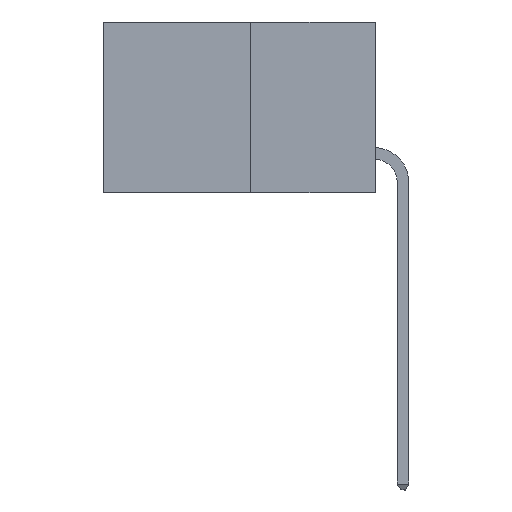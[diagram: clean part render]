
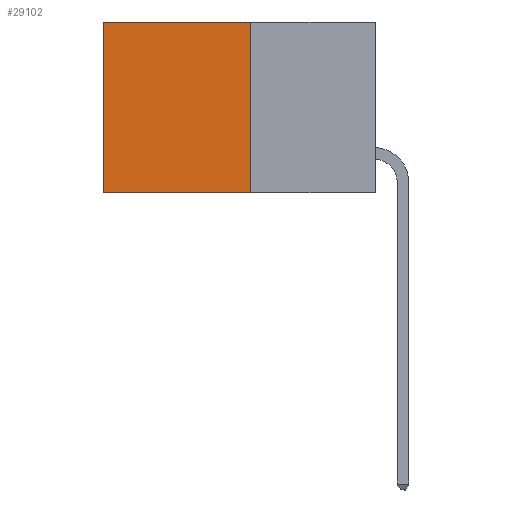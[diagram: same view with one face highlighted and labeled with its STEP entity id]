
A CAD part, left-side view. The second image highlights one B-rep face of the part: STEP entity #29102.
In plain terms, the highlighted planar face has unit normal (-1, 0, 0).
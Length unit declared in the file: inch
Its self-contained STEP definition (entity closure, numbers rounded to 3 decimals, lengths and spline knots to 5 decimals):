
#975 = VECTOR ( 'NONE', #7875, 39.37008 ) ;
#1063 = CARTESIAN_POINT ( 'NONE',  ( 0.277, 0.59, -0.37 ) ) ;
#1891 = CARTESIAN_POINT ( 'NONE',  ( 0.277, 0.27, -0.37 ) ) ;
#3534 = CARTESIAN_POINT ( 'NONE',  ( 0.277, 0.27, 0. ) ) ;
#4272 = DIRECTION ( 'NONE',  ( 1., 0., 0. ) ) ;
#5328 = FACE_OUTER_BOUND ( 'NONE', #15269, .T. ) ;
#5579 = EDGE_CURVE ( 'NONE', #9279, #24971, #29126, .T. ) ;
#6140 = EDGE_CURVE ( 'NONE', #8766, #24971, #7004, .T. ) ;
#6614 = CARTESIAN_POINT ( 'NONE',  ( 0.277, 0.59, -0.37 ) ) ;
#6671 = VECTOR ( 'NONE', #14795, 39.37008 ) ;
#7004 = LINE ( 'NONE', #19068, #975 ) ;
#7298 = CARTESIAN_POINT ( 'NONE',  ( 0.277, 0.59, 0. ) ) ;
#7875 = DIRECTION ( 'NONE',  ( 0., 1., 0. ) ) ;
#8153 = ORIENTED_EDGE ( 'NONE', *, *, #5579, .T. ) ;
#8766 = VERTEX_POINT ( 'NONE', #27818 ) ;
#9254 = ORIENTED_EDGE ( 'NONE', *, *, #22810, .T. ) ;
#9275 = CARTESIAN_POINT ( 'NONE',  ( 0.277, 0.27, -0.37 ) ) ;
#9279 = VERTEX_POINT ( 'NONE', #7298 ) ;
#11557 = DIRECTION ( 'NONE',  ( 0., 0., -1. ) ) ;
#14795 = DIRECTION ( 'NONE',  ( 0., 1., 0. ) ) ;
#15269 = EDGE_LOOP ( 'NONE', ( #8153, #20236, #20645, #9254 ) ) ;
#16528 = VECTOR ( 'NONE', #21336, 39.37008 ) ;
#17738 = CARTESIAN_POINT ( 'NONE',  ( 0.277, 0.27, 0. ) ) ;
#19068 = CARTESIAN_POINT ( 'NONE',  ( 0.277, 0.27, -0.37 ) ) ;
#20004 = DIRECTION ( 'NONE',  ( 0., 0., -1. ) ) ;
#20236 = ORIENTED_EDGE ( 'NONE', *, *, #6140, .F. ) ;
#20645 = ORIENTED_EDGE ( 'NONE', *, *, #27078, .F. ) ;
#21336 = DIRECTION ( 'NONE',  ( 0., 0., -1. ) ) ;
#22173 = VECTOR ( 'NONE', #11557, 39.37008 ) ;
#22810 = EDGE_CURVE ( 'NONE', #24274, #9279, #23858, .T. ) ;
#22877 = LINE ( 'NONE', #9275, #22173 ) ;
#23858 = LINE ( 'NONE', #3534, #6671 ) ;
#24274 = VERTEX_POINT ( 'NONE', #17738 ) ;
#24971 = VERTEX_POINT ( 'NONE', #6614 ) ;
#26813 = AXIS2_PLACEMENT_3D ( 'NONE', #1891, #4272, #20004 ) ;
#27078 = EDGE_CURVE ( 'NONE', #24274, #8766, #22877, .T. ) ;
#27818 = CARTESIAN_POINT ( 'NONE',  ( 0.277, 0.27, -0.37 ) ) ;
#28903 = PLANE ( 'NONE',  #26813 ) ;
#29102 = ADVANCED_FACE ( 'NONE', ( #5328 ), #28903, .F. ) ;
#29126 = LINE ( 'NONE', #1063, #16528 ) ;
